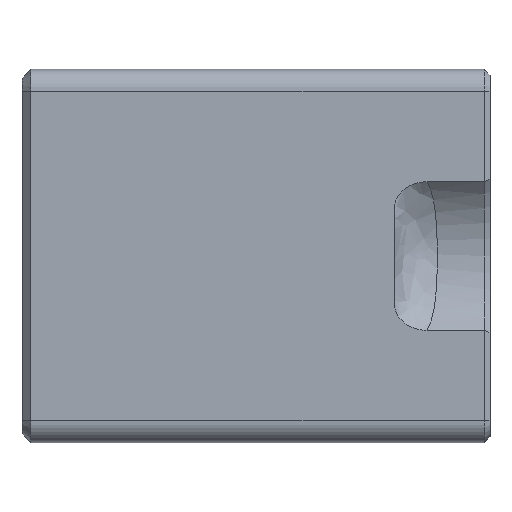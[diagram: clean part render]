
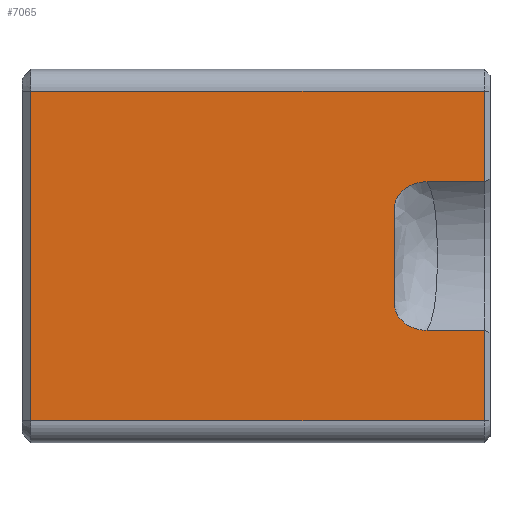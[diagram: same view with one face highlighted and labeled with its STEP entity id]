
A CAD part, front view. The second image highlights one B-rep face of the part: STEP entity #7065.
In plain terms, the highlighted planar face has unit normal (0, -1, 0).
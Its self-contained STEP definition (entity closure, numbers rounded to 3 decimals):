
#620=B_SPLINE_CURVE_WITH_KNOTS('',3,(#16668,#16669,#16670,#16671,#16672,
#16673,#16674,#16675,#16676,#16677,#16678,#16679,#16680,#16681,#16682,#16683,
#16684,#16685,#16686,#16687),.UNSPECIFIED.,.F.,.F.,(4,2,2,2,2,2,2,2,2,4),
(0.,0.,0.,0.002,0.007,
0.018,0.04,0.085,0.157,
0.234),.UNSPECIFIED.);
#621=B_SPLINE_CURVE_WITH_KNOTS('',3,(#16691,#16692,#16693,#16694,#16695,
#16696,#16697,#16698,#16699,#16700,#16701,#16702,#16703,#16704,#16705,#16706,
#16707,#16708,#16709,#16710),.UNSPECIFIED.,.F.,.F.,(4,2,2,2,2,2,2,2,2,4),
(0.,0.102,0.197,0.257,0.286,
0.3,0.306,0.31,0.31,
0.31),.UNSPECIFIED.);
#790=PLANE('',#7630);
#1260=FACE_OUTER_BOUND('',#1699,.T.);
#1699=EDGE_LOOP('',(#6402,#6403,#6404,#6405,#6406,#6407,#6408,#6409,#6410,
#6411));
#2095=LINE('',#16635,#2484);
#2104=LINE('',#16657,#2493);
#2105=LINE('',#16662,#2494);
#2106=LINE('',#16666,#2495);
#2107=LINE('',#16689,#2496);
#2108=LINE('',#16711,#2497);
#2109=LINE('',#16713,#2498);
#2110=LINE('',#16714,#2499);
#2484=VECTOR('',#8952,10.);
#2493=VECTOR('',#8985,10.);
#2494=VECTOR('',#8992,10.);
#2495=VECTOR('',#8997,10.);
#2496=VECTOR('',#8998,10.);
#2497=VECTOR('',#8999,10.);
#2498=VECTOR('',#9000,10.);
#2499=VECTOR('',#9001,10.);
#3393=VERTEX_POINT('',#16622);
#3394=VERTEX_POINT('',#16627);
#3395=VERTEX_POINT('',#16634);
#3396=VERTEX_POINT('',#16653);
#3397=VERTEX_POINT('',#16661);
#3398=VERTEX_POINT('',#16665);
#3399=VERTEX_POINT('',#16667);
#3400=VERTEX_POINT('',#16688);
#3401=VERTEX_POINT('',#16690);
#3402=VERTEX_POINT('',#16712);
#4397=EDGE_CURVE('',#3394,#3395,#2095,.T.);
#4410=EDGE_CURVE('',#3396,#3393,#2104,.T.);
#4412=EDGE_CURVE('',#3395,#3397,#2105,.T.);
#4414=EDGE_CURVE('',#3394,#3398,#2106,.T.);
#4415=EDGE_CURVE('',#3399,#3398,#620,.T.);
#4416=EDGE_CURVE('',#3399,#3400,#2107,.T.);
#4417=EDGE_CURVE('',#3400,#3401,#621,.F.);
#4418=EDGE_CURVE('',#3401,#3393,#2108,.T.);
#4419=EDGE_CURVE('',#3402,#3396,#2109,.T.);
#4420=EDGE_CURVE('',#3397,#3402,#2110,.T.);
#6402=ORIENTED_EDGE('',*,*,#4397,.F.);
#6403=ORIENTED_EDGE('',*,*,#4414,.T.);
#6404=ORIENTED_EDGE('',*,*,#4415,.F.);
#6405=ORIENTED_EDGE('',*,*,#4416,.T.);
#6406=ORIENTED_EDGE('',*,*,#4417,.T.);
#6407=ORIENTED_EDGE('',*,*,#4418,.T.);
#6408=ORIENTED_EDGE('',*,*,#4410,.F.);
#6409=ORIENTED_EDGE('',*,*,#4419,.F.);
#6410=ORIENTED_EDGE('',*,*,#4420,.F.);
#6411=ORIENTED_EDGE('',*,*,#4412,.F.);
#7065=ADVANCED_FACE('',(#1260),#790,.T.);
#7630=AXIS2_PLACEMENT_3D('',#16664,#8995,#8996);
#8952=DIRECTION('',(0.,0.,-1.));
#8985=DIRECTION('',(0.,0.,-1.));
#8992=DIRECTION('',(-1.,0.,0.));
#8995=DIRECTION('center_axis',(0.,-1.,0.));
#8996=DIRECTION('ref_axis',(0.,0.,1.));
#8997=DIRECTION('',(-1.,0.,0.));
#8998=DIRECTION('',(0.,0.,1.));
#8999=DIRECTION('',(1.,0.,0.));
#9000=DIRECTION('',(1.,0.,0.));
#9001=DIRECTION('',(0.,0.,1.));
#16622=CARTESIAN_POINT('',(-183.534,-11.455,5.083));
#16627=CARTESIAN_POINT('',(-183.534,-11.455,-5.083));
#16634=CARTESIAN_POINT('',(-183.534,-11.455,-11.264));
#16635=CARTESIAN_POINT('',(-183.534,-11.455,-6.128));
#16653=CARTESIAN_POINT('',(-183.534,-11.455,11.264));
#16657=CARTESIAN_POINT('',(-183.534,-11.455,-6.128));
#16661=CARTESIAN_POINT('',(-214.534,-11.455,-11.264));
#16662=CARTESIAN_POINT('',(-183.134,-11.455,-11.264));
#16664=CARTESIAN_POINT('Origin',(-183.134,-11.455,-12.256));
#16665=CARTESIAN_POINT('',(-187.44,-11.455,-5.083));
#16666=CARTESIAN_POINT('',(-183.134,-11.455,-5.083));
#16667=CARTESIAN_POINT('',(-189.634,-11.455,-3.546));
#16668=CARTESIAN_POINT('Ctrl Pts',(-189.634,-11.455,-3.546));
#16669=CARTESIAN_POINT('Ctrl Pts',(-189.634,-11.455,-3.546));
#16670=CARTESIAN_POINT('Ctrl Pts',(-189.634,-11.455,-3.547));
#16671=CARTESIAN_POINT('Ctrl Pts',(-189.634,-11.455,-3.548));
#16672=CARTESIAN_POINT('Ctrl Pts',(-189.634,-11.455,-3.549));
#16673=CARTESIAN_POINT('Ctrl Pts',(-189.634,-11.455,-3.558));
#16674=CARTESIAN_POINT('Ctrl Pts',(-189.633,-11.455,-3.566));
#16675=CARTESIAN_POINT('Ctrl Pts',(-189.63,-11.455,-3.592));
#16676=CARTESIAN_POINT('Ctrl Pts',(-189.627,-11.455,-3.61));
#16677=CARTESIAN_POINT('Ctrl Pts',(-189.616,-11.455,-3.667));
#16678=CARTESIAN_POINT('Ctrl Pts',(-189.605,-11.455,-3.707));
#16679=CARTESIAN_POINT('Ctrl Pts',(-189.566,-11.455,-3.826));
#16680=CARTESIAN_POINT('Ctrl Pts',(-189.531,-11.455,-3.905));
#16681=CARTESIAN_POINT('Ctrl Pts',(-189.407,-11.455,-4.136));
#16682=CARTESIAN_POINT('Ctrl Pts',(-189.297,-11.455,
-4.279));
#16683=CARTESIAN_POINT('Ctrl Pts',(-188.973,-11.455,
-4.603));
#16684=CARTESIAN_POINT('Ctrl Pts',(-188.724,-11.455,-4.771));
#16685=CARTESIAN_POINT('Ctrl Pts',(-188.119,-11.455,-5.02));
#16686=CARTESIAN_POINT('Ctrl Pts',(-187.781,-11.455,-5.083));
#16687=CARTESIAN_POINT('Ctrl Pts',(-187.44,-11.455,-5.083));
#16688=CARTESIAN_POINT('',(-189.634,-11.455,3.546));
#16689=CARTESIAN_POINT('',(-189.634,-11.455,-6.128));
#16690=CARTESIAN_POINT('',(-187.44,-11.455,5.083));
#16691=CARTESIAN_POINT('Ctrl Pts',(-187.44,-11.455,5.083));
#16692=CARTESIAN_POINT('Ctrl Pts',(-187.781,-11.455,5.083));
#16693=CARTESIAN_POINT('Ctrl Pts',(-188.119,-11.455,5.02));
#16694=CARTESIAN_POINT('Ctrl Pts',(-188.724,-11.455,4.771));
#16695=CARTESIAN_POINT('Ctrl Pts',(-188.973,-11.455,
4.603));
#16696=CARTESIAN_POINT('Ctrl Pts',(-189.297,-11.455,
4.279));
#16697=CARTESIAN_POINT('Ctrl Pts',(-189.407,-11.455,4.136));
#16698=CARTESIAN_POINT('Ctrl Pts',(-189.531,-11.455,3.905));
#16699=CARTESIAN_POINT('Ctrl Pts',(-189.566,-11.455,3.826));
#16700=CARTESIAN_POINT('Ctrl Pts',(-189.605,-11.455,3.707));
#16701=CARTESIAN_POINT('Ctrl Pts',(-189.616,-11.455,3.667));
#16702=CARTESIAN_POINT('Ctrl Pts',(-189.627,-11.455,3.61));
#16703=CARTESIAN_POINT('Ctrl Pts',(-189.63,-11.455,3.592));
#16704=CARTESIAN_POINT('Ctrl Pts',(-189.633,-11.455,3.565));
#16705=CARTESIAN_POINT('Ctrl Pts',(-189.634,-11.455,3.557));
#16706=CARTESIAN_POINT('Ctrl Pts',(-189.634,-11.455,3.549));
#16707=CARTESIAN_POINT('Ctrl Pts',(-189.634,-11.455,3.548));
#16708=CARTESIAN_POINT('Ctrl Pts',(-189.634,-11.455,3.547));
#16709=CARTESIAN_POINT('Ctrl Pts',(-189.634,-11.455,3.546));
#16710=CARTESIAN_POINT('Ctrl Pts',(-189.634,-11.455,3.546));
#16711=CARTESIAN_POINT('',(-183.134,-11.455,5.083));
#16712=CARTESIAN_POINT('',(-214.534,-11.455,11.264));
#16713=CARTESIAN_POINT('',(-183.134,-11.455,11.264));
#16714=CARTESIAN_POINT('',(-214.534,-11.455,-6.128));
